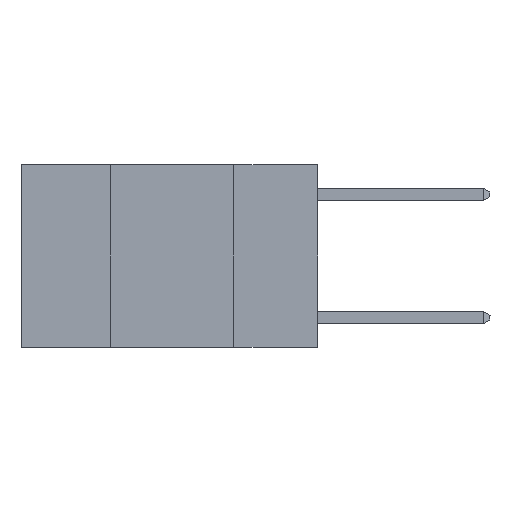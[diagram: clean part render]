
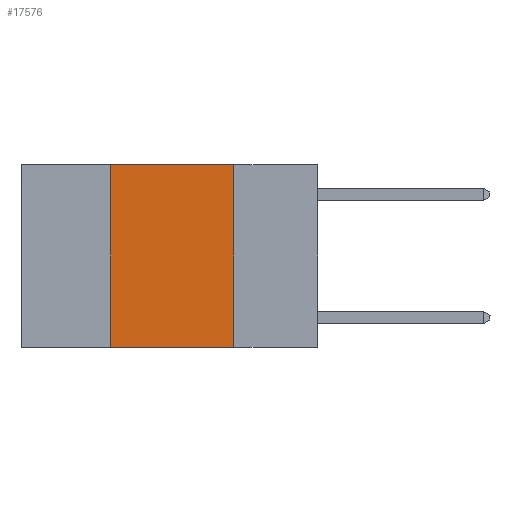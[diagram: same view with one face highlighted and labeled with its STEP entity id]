
A CAD part, left-side view. The second image highlights one B-rep face of the part: STEP entity #17576.
In plain terms, the highlighted planar face has unit normal (-1, 0, 0).
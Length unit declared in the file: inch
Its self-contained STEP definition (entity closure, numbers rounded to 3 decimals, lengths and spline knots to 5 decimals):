
#270 = EDGE_LOOP ( 'NONE', ( #19112, #19166, #20273, #20315 ) ) ;
#712 = CARTESIAN_POINT ( 'NONE',  ( 0., 0.17, 0. ) ) ;
#728 = LINE ( 'NONE', #18394, #4723 ) ;
#1561 = EDGE_CURVE ( 'NONE', #20519, #14858, #728, .T. ) ;
#2328 = LINE ( 'NONE', #21789, #15484 ) ;
#2420 = DIRECTION ( 'NONE',  ( 0., 0., -1. ) ) ;
#3037 = VERTEX_POINT ( 'NONE', #10398 ) ;
#3094 = DIRECTION ( 'NONE',  ( 0., -1., 0. ) ) ;
#4723 = VECTOR ( 'NONE', #20154, 39.37008 ) ;
#5447 = AXIS2_PLACEMENT_3D ( 'NONE', #17435, #5508, #17498 ) ;
#5508 = DIRECTION ( 'NONE',  ( 1., 0., 0. ) ) ;
#6376 = LINE ( 'NONE', #712, #14943 ) ;
#8787 = EDGE_CURVE ( 'NONE', #21630, #3037, #6376, .T. ) ;
#9533 = LINE ( 'NONE', #10143, #13541 ) ;
#10143 = CARTESIAN_POINT ( 'NONE',  ( 0., 0.6, -0.37 ) ) ;
#10398 = CARTESIAN_POINT ( 'NONE',  ( 0., 0.17, -0.37 ) ) ;
#11167 = CARTESIAN_POINT ( 'NONE',  ( 0., 0.42, -0.37 ) ) ;
#11859 = EDGE_CURVE ( 'NONE', #14858, #21630, #2328, .T. ) ;
#13541 = VECTOR ( 'NONE', #20355, 39.37008 ) ;
#14507 = CARTESIAN_POINT ( 'NONE',  ( 0., 0.42, 0. ) ) ;
#14858 = VERTEX_POINT ( 'NONE', #14507 ) ;
#14943 = VECTOR ( 'NONE', #2420, 39.37008 ) ;
#15484 = VECTOR ( 'NONE', #3094, 39.37008 ) ;
#15773 = PLANE ( 'NONE',  #5447 ) ;
#17435 = CARTESIAN_POINT ( 'NONE',  ( 0., 0.6, 0. ) ) ;
#17498 = DIRECTION ( 'NONE',  ( 0., 0., -1. ) ) ;
#17576 = ADVANCED_FACE ( 'NONE', ( #18234 ), #15773, .F. ) ;
#18234 = FACE_OUTER_BOUND ( 'NONE', #270, .T. ) ;
#18394 = CARTESIAN_POINT ( 'NONE',  ( 0., 0.42, 0. ) ) ;
#19112 = ORIENTED_EDGE ( 'NONE', *, *, #8787, .F. ) ;
#19166 = ORIENTED_EDGE ( 'NONE', *, *, #11859, .F. ) ;
#19331 = CARTESIAN_POINT ( 'NONE',  ( 0., 0.17, 0. ) ) ;
#20154 = DIRECTION ( 'NONE',  ( 0., 0., 1. ) ) ;
#20273 = ORIENTED_EDGE ( 'NONE', *, *, #1561, .F. ) ;
#20315 = ORIENTED_EDGE ( 'NONE', *, *, #21403, .T. ) ;
#20355 = DIRECTION ( 'NONE',  ( 0., -1., 0. ) ) ;
#20519 = VERTEX_POINT ( 'NONE', #11167 ) ;
#21403 = EDGE_CURVE ( 'NONE', #20519, #3037, #9533, .T. ) ;
#21630 = VERTEX_POINT ( 'NONE', #19331 ) ;
#21789 = CARTESIAN_POINT ( 'NONE',  ( 0., 0.6, 0. ) ) ;
